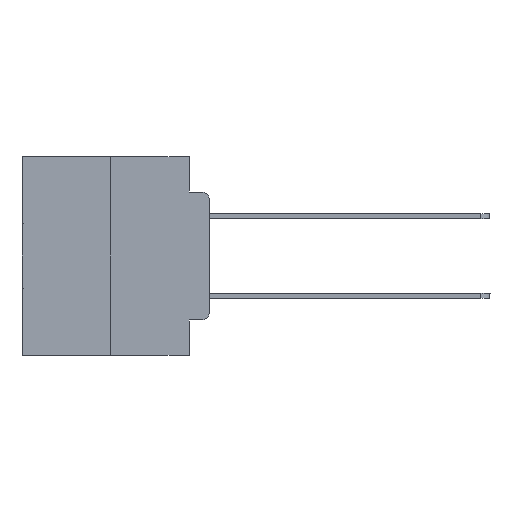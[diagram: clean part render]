
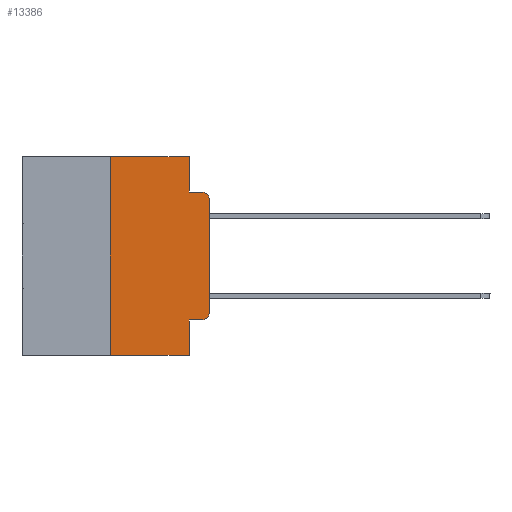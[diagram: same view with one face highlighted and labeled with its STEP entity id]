
A CAD part, left-side view. The second image highlights one B-rep face of the part: STEP entity #13386.
In plain terms, the highlighted planar face has unit normal (-1, 0, 0).
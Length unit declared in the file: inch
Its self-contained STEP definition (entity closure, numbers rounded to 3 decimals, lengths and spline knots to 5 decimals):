
#370 = DIRECTION ( 'NONE',  ( 0., 0., -1. ) ) ;
#695 = CARTESIAN_POINT ( 'NONE',  ( 0., 0.051, 0. ) ) ;
#1265 = EDGE_LOOP ( 'NONE', ( #29240, #13509, #6078, #13833, #10654, #13636, #9652, #18830, #8671, #10579 ) ) ;
#1583 = DIRECTION ( 'NONE',  ( 0., -1., 0. ) ) ;
#1789 = LINE ( 'NONE', #17520, #27964 ) ;
#2085 = LINE ( 'NONE', #17959, #26008 ) ;
#2384 = DIRECTION ( 'NONE',  ( 0., -1., 0. ) ) ;
#2899 = CARTESIAN_POINT ( 'NONE',  ( 0., 0.02, -0.3915 ) ) ;
#3588 = EDGE_CURVE ( 'NONE', #14347, #13129, #24670, .T. ) ;
#3872 = DIRECTION ( 'NONE',  ( 0., 0., 1. ) ) ;
#4940 = DIRECTION ( 'NONE',  ( -1., 0., 0. ) ) ;
#5605 = VECTOR ( 'NONE', #6976, 39.37008 ) ;
#6078 = ORIENTED_EDGE ( 'NONE', *, *, #25231, .F. ) ;
#6317 = EDGE_CURVE ( 'NONE', #19009, #28984, #15721, .T. ) ;
#6390 = EDGE_CURVE ( 'NONE', #19009, #13129, #2085, .T. ) ;
#6593 = FACE_OUTER_BOUND ( 'NONE', #1265, .T. ) ;
#6866 = EDGE_CURVE ( 'NONE', #7631, #13618, #22245, .T. ) ;
#6941 = CARTESIAN_POINT ( 'NONE',  ( 0., 0.051, 0. ) ) ;
#6976 = DIRECTION ( 'NONE',  ( 0., 0., 1. ) ) ;
#6981 = CARTESIAN_POINT ( 'NONE',  ( 0., 0.02, -0.4115 ) ) ;
#7337 = EDGE_CURVE ( 'NONE', #16488, #14713, #17307, .T. ) ;
#7607 = DIRECTION ( 'NONE',  ( 0., 0., -1. ) ) ;
#7631 = VERTEX_POINT ( 'NONE', #6981 ) ;
#8050 = CARTESIAN_POINT ( 'NONE',  ( 0., 0., -0.3915 ) ) ;
#8671 = ORIENTED_EDGE ( 'NONE', *, *, #21839, .T. ) ;
#8879 = CARTESIAN_POINT ( 'NONE',  ( 0., 0.25, 0. ) ) ;
#9429 = AXIS2_PLACEMENT_3D ( 'NONE', #2899, #14018, #370 ) ;
#9483 = VERTEX_POINT ( 'NONE', #21935 ) ;
#9652 = ORIENTED_EDGE ( 'NONE', *, *, #6390, .T. ) ;
#10069 = VECTOR ( 'NONE', #23144, 39.37008 ) ;
#10262 = DIRECTION ( 'NONE',  ( 0., 0., -1. ) ) ;
#10579 = ORIENTED_EDGE ( 'NONE', *, *, #6866, .T. ) ;
#10654 = ORIENTED_EDGE ( 'NONE', *, *, #13665, .F. ) ;
#11758 = CARTESIAN_POINT ( 'NONE',  ( 0., 0., -0.1085 ) ) ;
#11763 = CARTESIAN_POINT ( 'NONE',  ( 0., 0.473, 0. ) ) ;
#13129 = VERTEX_POINT ( 'NONE', #19803 ) ;
#13386 = ADVANCED_FACE ( 'NONE', ( #6593 ), #15626, .F. ) ;
#13509 = ORIENTED_EDGE ( 'NONE', *, *, #7337, .T. ) ;
#13618 = VERTEX_POINT ( 'NONE', #8050 ) ;
#13636 = ORIENTED_EDGE ( 'NONE', *, *, #6317, .F. ) ;
#13665 = EDGE_CURVE ( 'NONE', #28984, #29216, #17602, .T. ) ;
#13833 = ORIENTED_EDGE ( 'NONE', *, *, #29150, .F. ) ;
#13854 = CARTESIAN_POINT ( 'NONE',  ( 0., 0.02, -0.0885 ) ) ;
#14018 = DIRECTION ( 'NONE',  ( -1., 0., 0. ) ) ;
#14329 = DIRECTION ( 'NONE',  ( 0., -1., 0. ) ) ;
#14347 = VERTEX_POINT ( 'NONE', #23832 ) ;
#14517 = VECTOR ( 'NONE', #15834, 39.37008 ) ;
#14713 = VERTEX_POINT ( 'NONE', #13854 ) ;
#15366 = EDGE_CURVE ( 'NONE', #13618, #16488, #1789, .T. ) ;
#15626 = PLANE ( 'NONE',  #16027 ) ;
#15721 = LINE ( 'NONE', #24929, #5605 ) ;
#15755 = CARTESIAN_POINT ( 'NONE',  ( 0., 0.051, 0. ) ) ;
#15834 = DIRECTION ( 'NONE',  ( 0., 0., -1. ) ) ;
#16027 = AXIS2_PLACEMENT_3D ( 'NONE', #11763, #23349, #7607 ) ;
#16488 = VERTEX_POINT ( 'NONE', #11758 ) ;
#16554 = LINE ( 'NONE', #25619, #22307 ) ;
#17307 = CIRCLE ( 'NONE', #19672, 0.02 ) ;
#17520 = CARTESIAN_POINT ( 'NONE',  ( 0., 0., 0. ) ) ;
#17602 = LINE ( 'NONE', #21925, #20216 ) ;
#17758 = CARTESIAN_POINT ( 'NONE',  ( 0., 0.25, -0.5 ) ) ;
#17959 = CARTESIAN_POINT ( 'NONE',  ( 0., 0.473, -0.5 ) ) ;
#18532 = LINE ( 'NONE', #27293, #10069 ) ;
#18830 = ORIENTED_EDGE ( 'NONE', *, *, #3588, .F. ) ;
#19009 = VERTEX_POINT ( 'NONE', #17758 ) ;
#19672 = AXIS2_PLACEMENT_3D ( 'NONE', #25273, #4940, #10262 ) ;
#19803 = CARTESIAN_POINT ( 'NONE',  ( 0., 0.051, -0.5 ) ) ;
#20216 = VECTOR ( 'NONE', #1583, 39.37008 ) ;
#21839 = EDGE_CURVE ( 'NONE', #14347, #7631, #16554, .T. ) ;
#21925 = CARTESIAN_POINT ( 'NONE',  ( 0., 0.473, 0. ) ) ;
#21935 = CARTESIAN_POINT ( 'NONE',  ( 0., 0.051, -0.0885 ) ) ;
#22245 = CIRCLE ( 'NONE', #9429, 0.02 ) ;
#22307 = VECTOR ( 'NONE', #14329, 39.37008 ) ;
#23144 = DIRECTION ( 'NONE',  ( 0., -1., 0. ) ) ;
#23349 = DIRECTION ( 'NONE',  ( 1., 0., 0. ) ) ;
#23787 = VECTOR ( 'NONE', #24822, 39.37008 ) ;
#23832 = CARTESIAN_POINT ( 'NONE',  ( 0., 0.051, -0.4115 ) ) ;
#24670 = LINE ( 'NONE', #15755, #23787 ) ;
#24822 = DIRECTION ( 'NONE',  ( 0., 0., -1. ) ) ;
#24929 = CARTESIAN_POINT ( 'NONE',  ( 0., 0.25, 0. ) ) ;
#25231 = EDGE_CURVE ( 'NONE', #9483, #14713, #18532, .T. ) ;
#25273 = CARTESIAN_POINT ( 'NONE',  ( 0., 0.02, -0.1085 ) ) ;
#25619 = CARTESIAN_POINT ( 'NONE',  ( 0., 0.051, -0.4115 ) ) ;
#26008 = VECTOR ( 'NONE', #2384, 39.37008 ) ;
#27272 = LINE ( 'NONE', #6941, #14517 ) ;
#27293 = CARTESIAN_POINT ( 'NONE',  ( 0., 0.051, -0.0885 ) ) ;
#27964 = VECTOR ( 'NONE', #3872, 39.37008 ) ;
#28984 = VERTEX_POINT ( 'NONE', #8879 ) ;
#29150 = EDGE_CURVE ( 'NONE', #29216, #9483, #27272, .T. ) ;
#29216 = VERTEX_POINT ( 'NONE', #695 ) ;
#29240 = ORIENTED_EDGE ( 'NONE', *, *, #15366, .T. ) ;
